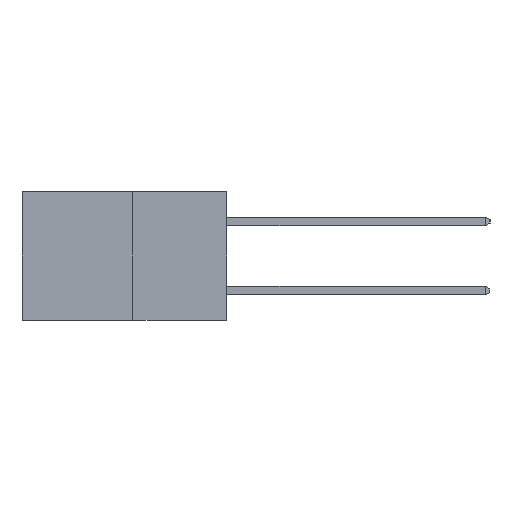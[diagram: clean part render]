
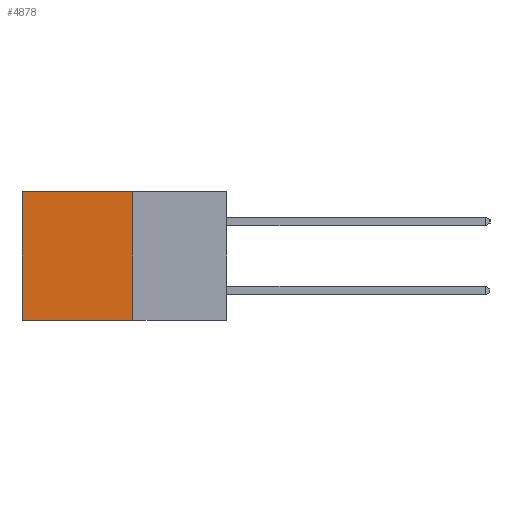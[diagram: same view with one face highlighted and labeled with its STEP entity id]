
A CAD part, left-side view. The second image highlights one B-rep face of the part: STEP entity #4878.
In plain terms, the highlighted planar face has unit normal (-1, 0, 0).
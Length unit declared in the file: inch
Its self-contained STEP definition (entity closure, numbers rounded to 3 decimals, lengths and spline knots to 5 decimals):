
#160 = DIRECTION ( 'NONE',  ( 0., 1., 0. ) ) ;
#485 = DIRECTION ( 'NONE',  ( 0., 1., 0. ) ) ;
#533 = CARTESIAN_POINT ( 'NONE',  ( 0.277, 0.27, -0.37 ) ) ;
#1130 = ORIENTED_EDGE ( 'NONE', *, *, #7896, .T. ) ;
#1709 = VECTOR ( 'NONE', #7406, 39.37008 ) ;
#2794 = VERTEX_POINT ( 'NONE', #4584 ) ;
#3267 = DIRECTION ( 'NONE',  ( 0., 0., -1. ) ) ;
#3316 = DIRECTION ( 'NONE',  ( 1., 0., 0. ) ) ;
#3399 = CARTESIAN_POINT ( 'NONE',  ( 0.277, 0.27, -0.37 ) ) ;
#3576 = PLANE ( 'NONE',  #4281 ) ;
#3625 = CARTESIAN_POINT ( 'NONE',  ( 0.277, 0.27, -0.37 ) ) ;
#3648 = LINE ( 'NONE', #7421, #1709 ) ;
#4147 = EDGE_CURVE ( 'NONE', #8306, #8541, #3648, .T. ) ;
#4281 = AXIS2_PLACEMENT_3D ( 'NONE', #3625, #3316, #3267 ) ;
#4415 = VECTOR ( 'NONE', #485, 39.37008 ) ;
#4443 = LINE ( 'NONE', #4972, #8313 ) ;
#4584 = CARTESIAN_POINT ( 'NONE',  ( 0.277, 0.59, 0. ) ) ;
#4648 = LINE ( 'NONE', #7147, #4415 ) ;
#4834 = CARTESIAN_POINT ( 'NONE',  ( 0.277, 0.59, -0.37 ) ) ;
#4878 = ADVANCED_FACE ( 'NONE', ( #7928 ), #3576, .F. ) ;
#4961 = VECTOR ( 'NONE', #160, 39.37008 ) ;
#4972 = CARTESIAN_POINT ( 'NONE',  ( 0.277, 0.59, -0.37 ) ) ;
#5196 = EDGE_CURVE ( 'NONE', #8541, #5768, #6940, .T. ) ;
#5379 = ORIENTED_EDGE ( 'NONE', *, *, #9354, .T. ) ;
#5768 = VERTEX_POINT ( 'NONE', #4834 ) ;
#6427 = EDGE_LOOP ( 'NONE', ( #1130, #7077, #8910, #5379 ) ) ;
#6493 = DIRECTION ( 'NONE',  ( 0., 0., -1. ) ) ;
#6940 = LINE ( 'NONE', #533, #4961 ) ;
#7077 = ORIENTED_EDGE ( 'NONE', *, *, #5196, .F. ) ;
#7147 = CARTESIAN_POINT ( 'NONE',  ( 0.277, 0.27, 0. ) ) ;
#7406 = DIRECTION ( 'NONE',  ( 0., 0., -1. ) ) ;
#7421 = CARTESIAN_POINT ( 'NONE',  ( 0.277, 0.27, -0.37 ) ) ;
#7896 = EDGE_CURVE ( 'NONE', #2794, #5768, #4443, .T. ) ;
#7928 = FACE_OUTER_BOUND ( 'NONE', #6427, .T. ) ;
#8306 = VERTEX_POINT ( 'NONE', #8964 ) ;
#8313 = VECTOR ( 'NONE', #6493, 39.37008 ) ;
#8541 = VERTEX_POINT ( 'NONE', #3399 ) ;
#8910 = ORIENTED_EDGE ( 'NONE', *, *, #4147, .F. ) ;
#8964 = CARTESIAN_POINT ( 'NONE',  ( 0.277, 0.27, 0. ) ) ;
#9354 = EDGE_CURVE ( 'NONE', #8306, #2794, #4648, .T. ) ;
